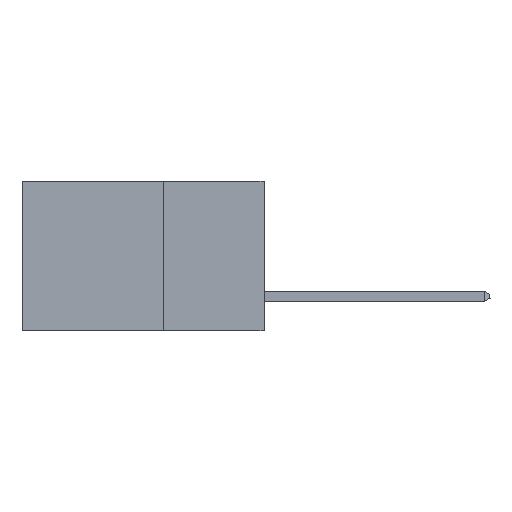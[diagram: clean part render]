
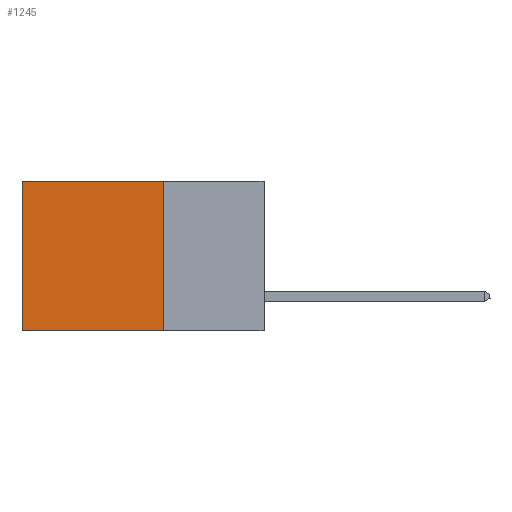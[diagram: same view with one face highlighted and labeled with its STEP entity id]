
A CAD part, left-side view. The second image highlights one B-rep face of the part: STEP entity #1245.
In plain terms, the highlighted planar face has unit normal (-1, 0, 0).
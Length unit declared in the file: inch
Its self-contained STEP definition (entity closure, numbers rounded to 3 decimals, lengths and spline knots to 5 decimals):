
#38 = DIRECTION ( 'NONE',  ( 1., 0., 0. ) ) ;
#1245 = ADVANCED_FACE ( 'NONE', ( #8602 ), #9535, .F. ) ;
#2135 = DIRECTION ( 'NONE',  ( 0., 0., -1. ) ) ;
#2824 = EDGE_CURVE ( 'NONE', #14288, #6170, #19614, .T. ) ;
#3094 = CARTESIAN_POINT ( 'NONE',  ( 0.298, 0.25, -0.37 ) ) ;
#5166 = EDGE_CURVE ( 'NONE', #9048, #6170, #9915, .T. ) ;
#5661 = AXIS2_PLACEMENT_3D ( 'NONE', #17551, #38, #12864 ) ;
#6132 = EDGE_CURVE ( 'NONE', #10448, #9048, #11961, .T. ) ;
#6170 = VERTEX_POINT ( 'NONE', #8675 ) ;
#6430 = DIRECTION ( 'NONE',  ( 0., 1., 0. ) ) ;
#6884 = EDGE_LOOP ( 'NONE', ( #14751, #14439, #19973, #14317 ) ) ;
#6919 = CARTESIAN_POINT ( 'NONE',  ( 0.298, 0.25, 0. ) ) ;
#7381 = CARTESIAN_POINT ( 'NONE',  ( 0.298, 0.25, -0.37 ) ) ;
#8396 = EDGE_CURVE ( 'NONE', #10448, #14288, #10067, .T. ) ;
#8602 = FACE_OUTER_BOUND ( 'NONE', #6884, .T. ) ;
#8675 = CARTESIAN_POINT ( 'NONE',  ( 0.298, 0.6, -0.37 ) ) ;
#9048 = VERTEX_POINT ( 'NONE', #7381 ) ;
#9161 = VECTOR ( 'NONE', #6430, 39.37008 ) ;
#9535 = PLANE ( 'NONE',  #5661 ) ;
#9915 = LINE ( 'NONE', #3094, #9161 ) ;
#10067 = LINE ( 'NONE', #18043, #18613 ) ;
#10448 = VERTEX_POINT ( 'NONE', #10915 ) ;
#10915 = CARTESIAN_POINT ( 'NONE',  ( 0.298, 0.25, 0. ) ) ;
#11961 = LINE ( 'NONE', #6919, #13725 ) ;
#12864 = DIRECTION ( 'NONE',  ( 0., 0., -1. ) ) ;
#13294 = DIRECTION ( 'NONE',  ( 0., 1., 0. ) ) ;
#13725 = VECTOR ( 'NONE', #16793, 39.37008 ) ;
#14288 = VERTEX_POINT ( 'NONE', #16135 ) ;
#14317 = ORIENTED_EDGE ( 'NONE', *, *, #8396, .T. ) ;
#14439 = ORIENTED_EDGE ( 'NONE', *, *, #5166, .F. ) ;
#14751 = ORIENTED_EDGE ( 'NONE', *, *, #2824, .T. ) ;
#16135 = CARTESIAN_POINT ( 'NONE',  ( 0.298, 0.6, 0. ) ) ;
#16793 = DIRECTION ( 'NONE',  ( 0., 0., -1. ) ) ;
#17551 = CARTESIAN_POINT ( 'NONE',  ( 0.298, 0.25, 0. ) ) ;
#18043 = CARTESIAN_POINT ( 'NONE',  ( 0.298, 0.25, 0. ) ) ;
#18110 = CARTESIAN_POINT ( 'NONE',  ( 0.298, 0.6, 0. ) ) ;
#18613 = VECTOR ( 'NONE', #13294, 39.37008 ) ;
#19614 = LINE ( 'NONE', #18110, #20122 ) ;
#19973 = ORIENTED_EDGE ( 'NONE', *, *, #6132, .F. ) ;
#20122 = VECTOR ( 'NONE', #2135, 39.37008 ) ;
